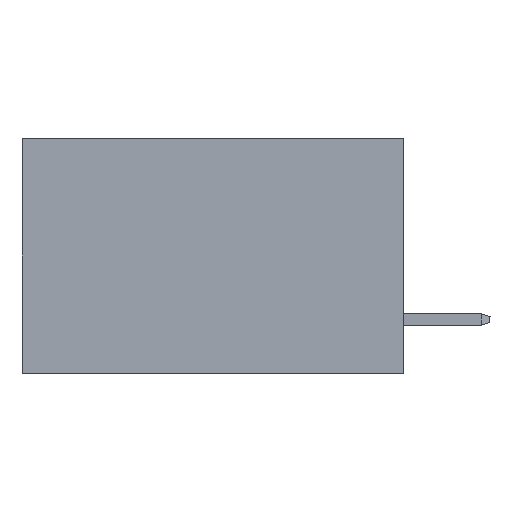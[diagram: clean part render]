
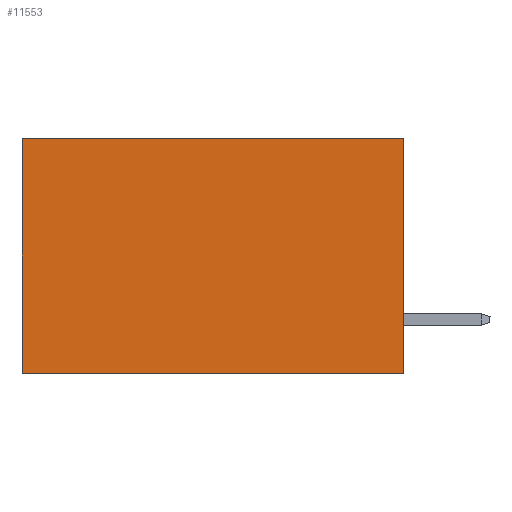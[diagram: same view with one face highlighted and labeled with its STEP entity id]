
A CAD part, left-side view. The second image highlights one B-rep face of the part: STEP entity #11553.
In plain terms, the highlighted planar face has unit normal (-1, 0, 0).
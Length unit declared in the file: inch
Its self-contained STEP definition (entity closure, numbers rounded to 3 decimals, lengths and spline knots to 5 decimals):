
#430 = ORIENTED_EDGE ( 'NONE', *, *, #31735, .F. ) ;
#487 = LINE ( 'NONE', #25417, #29582 ) ;
#489 = ORIENTED_EDGE ( 'NONE', *, *, #26839, .T. ) ;
#610 = DIRECTION ( 'NONE',  ( 0., 1., 0. ) ) ;
#636 = VERTEX_POINT ( 'NONE', #20977 ) ;
#1140 = EDGE_LOOP ( 'NONE', ( #30315, #5037, #430, #489 ) ) ;
#1476 = VERTEX_POINT ( 'NONE', #23019 ) ;
#2555 = VECTOR ( 'NONE', #610, 39.37008 ) ;
#3743 = PLANE ( 'NONE',  #26568 ) ;
#5037 = ORIENTED_EDGE ( 'NONE', *, *, #5809, .F. ) ;
#5809 = EDGE_CURVE ( 'NONE', #20051, #21121, #20656, .T. ) ;
#5971 = CARTESIAN_POINT ( 'NONE',  ( 0.2875, 0., 0. ) ) ;
#7569 = DIRECTION ( 'NONE',  ( 0., 1., 0. ) ) ;
#8748 = CARTESIAN_POINT ( 'NONE',  ( 0.2875, 0., 0. ) ) ;
#9637 = EDGE_CURVE ( 'NONE', #636, #21121, #487, .T. ) ;
#11553 = ADVANCED_FACE ( 'NONE', ( #16031 ), #3743, .F. ) ;
#11857 = VECTOR ( 'NONE', #18913, 39.37008 ) ;
#14078 = CARTESIAN_POINT ( 'NONE',  ( 0.2875, 0., -0.37 ) ) ;
#16031 = FACE_OUTER_BOUND ( 'NONE', #1140, .T. ) ;
#17280 = LINE ( 'NONE', #27163, #28353 ) ;
#18472 = DIRECTION ( 'NONE',  ( 1., 0., 0. ) ) ;
#18913 = DIRECTION ( 'NONE',  ( 0., 0., -1. ) ) ;
#20051 = VERTEX_POINT ( 'NONE', #14078 ) ;
#20656 = LINE ( 'NONE', #23101, #2555 ) ;
#20977 = CARTESIAN_POINT ( 'NONE',  ( 0.2875, 0.6, 0. ) ) ;
#21121 = VERTEX_POINT ( 'NONE', #29748 ) ;
#23019 = CARTESIAN_POINT ( 'NONE',  ( 0.2875, 0., 0. ) ) ;
#23101 = CARTESIAN_POINT ( 'NONE',  ( 0.2875, 0., -0.37 ) ) ;
#25417 = CARTESIAN_POINT ( 'NONE',  ( 0.2875, 0.6, 0. ) ) ;
#25749 = DIRECTION ( 'NONE',  ( 0., 0., -1. ) ) ;
#26568 = AXIS2_PLACEMENT_3D ( 'NONE', #8748, #18472, #28047 ) ;
#26839 = EDGE_CURVE ( 'NONE', #1476, #636, #17280, .T. ) ;
#27163 = CARTESIAN_POINT ( 'NONE',  ( 0.2875, 0., 0. ) ) ;
#28047 = DIRECTION ( 'NONE',  ( 0., 0., -1. ) ) ;
#28170 = LINE ( 'NONE', #5971, #11857 ) ;
#28353 = VECTOR ( 'NONE', #7569, 39.37008 ) ;
#29582 = VECTOR ( 'NONE', #25749, 39.37008 ) ;
#29748 = CARTESIAN_POINT ( 'NONE',  ( 0.2875, 0.6, -0.37 ) ) ;
#30315 = ORIENTED_EDGE ( 'NONE', *, *, #9637, .T. ) ;
#31735 = EDGE_CURVE ( 'NONE', #1476, #20051, #28170, .T. ) ;
